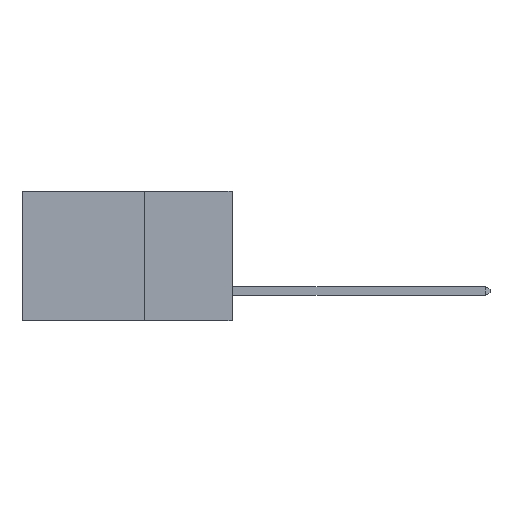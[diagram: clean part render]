
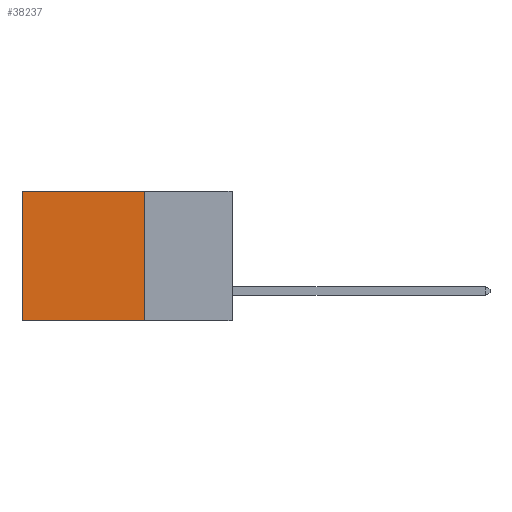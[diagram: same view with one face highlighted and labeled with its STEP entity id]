
A CAD part, left-side view. The second image highlights one B-rep face of the part: STEP entity #38237.
In plain terms, the highlighted planar face has unit normal (-1, 0, 0).
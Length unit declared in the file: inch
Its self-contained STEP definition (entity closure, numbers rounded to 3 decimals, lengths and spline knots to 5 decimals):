
#488 = AXIS2_PLACEMENT_3D ( 'NONE', #28459, #41474, #28748 ) ;
#2249 = CARTESIAN_POINT ( 'NONE',  ( 0.2875, 0.25, 0. ) ) ;
#2493 = ORIENTED_EDGE ( 'NONE', *, *, #35949, .F. ) ;
#3178 = PLANE ( 'NONE',  #488 ) ;
#7874 = VECTOR ( 'NONE', #13969, 39.37008 ) ;
#9683 = VECTOR ( 'NONE', #10627, 39.37008 ) ;
#10627 = DIRECTION ( 'NONE',  ( 0., 1., 0. ) ) ;
#11436 = EDGE_LOOP ( 'NONE', ( #19277, #41093, #2493, #15260 ) ) ;
#13969 = DIRECTION ( 'NONE',  ( 0., 1., 0. ) ) ;
#15260 = ORIENTED_EDGE ( 'NONE', *, *, #32254, .T. ) ;
#16114 = FACE_OUTER_BOUND ( 'NONE', #11436, .T. ) ;
#18837 = EDGE_CURVE ( 'NONE', #35442, #32876, #24078, .T. ) ;
#19277 = ORIENTED_EDGE ( 'NONE', *, *, #18837, .T. ) ;
#19312 = LINE ( 'NONE', #22627, #20320 ) ;
#20320 = VECTOR ( 'NONE', #25691, 39.37008 ) ;
#20527 = CARTESIAN_POINT ( 'NONE',  ( 0.2875, 0.25, -0.37 ) ) ;
#22627 = CARTESIAN_POINT ( 'NONE',  ( 0.2875, 0.25, 0. ) ) ;
#22740 = CARTESIAN_POINT ( 'NONE',  ( 0.2875, 0.25, -0.37 ) ) ;
#23380 = CARTESIAN_POINT ( 'NONE',  ( 0.2875, 0.25, 0. ) ) ;
#23746 = CARTESIAN_POINT ( 'NONE',  ( 0.2875, 0.6, -0.37 ) ) ;
#24078 = LINE ( 'NONE', #25952, #33571 ) ;
#25203 = LINE ( 'NONE', #23380, #9683 ) ;
#25691 = DIRECTION ( 'NONE',  ( 0., 0., -1. ) ) ;
#25952 = CARTESIAN_POINT ( 'NONE',  ( 0.2875, 0.6, 0. ) ) ;
#28231 = EDGE_CURVE ( 'NONE', #34629, #32876, #39898, .T. ) ;
#28459 = CARTESIAN_POINT ( 'NONE',  ( 0.2875, 0.25, 0. ) ) ;
#28748 = DIRECTION ( 'NONE',  ( 0., 0., -1. ) ) ;
#32233 = DIRECTION ( 'NONE',  ( 0., 0., -1. ) ) ;
#32254 = EDGE_CURVE ( 'NONE', #32505, #35442, #25203, .T. ) ;
#32505 = VERTEX_POINT ( 'NONE', #2249 ) ;
#32876 = VERTEX_POINT ( 'NONE', #23746 ) ;
#33571 = VECTOR ( 'NONE', #32233, 39.37008 ) ;
#34629 = VERTEX_POINT ( 'NONE', #22740 ) ;
#35442 = VERTEX_POINT ( 'NONE', #39528 ) ;
#35949 = EDGE_CURVE ( 'NONE', #32505, #34629, #19312, .T. ) ;
#38237 = ADVANCED_FACE ( 'NONE', ( #16114 ), #3178, .F. ) ;
#39528 = CARTESIAN_POINT ( 'NONE',  ( 0.2875, 0.6, 0. ) ) ;
#39898 = LINE ( 'NONE', #20527, #7874 ) ;
#41093 = ORIENTED_EDGE ( 'NONE', *, *, #28231, .F. ) ;
#41474 = DIRECTION ( 'NONE',  ( 1., 0., 0. ) ) ;
